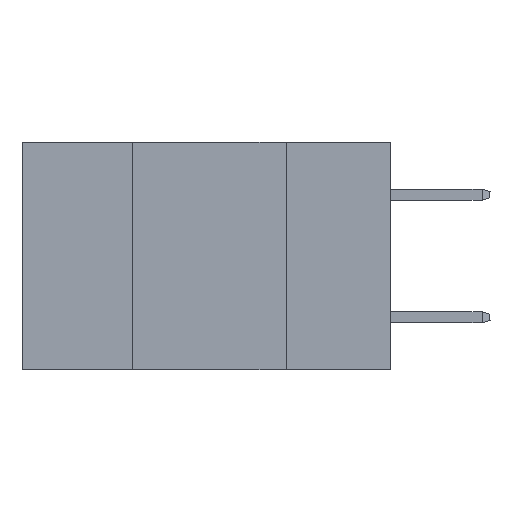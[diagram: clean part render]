
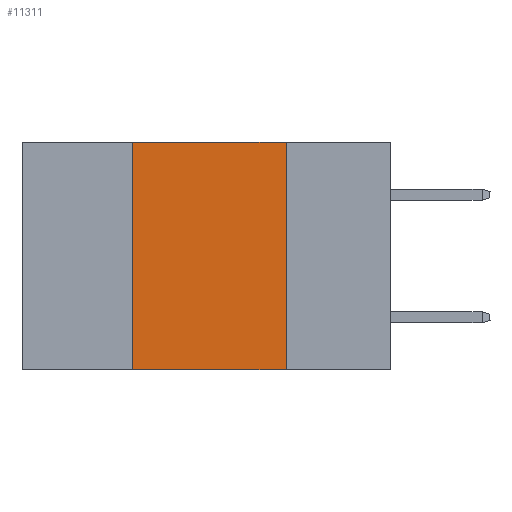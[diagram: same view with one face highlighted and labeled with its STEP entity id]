
A CAD part, left-side view. The second image highlights one B-rep face of the part: STEP entity #11311.
In plain terms, the highlighted planar face has unit normal (-1, 0, 0).
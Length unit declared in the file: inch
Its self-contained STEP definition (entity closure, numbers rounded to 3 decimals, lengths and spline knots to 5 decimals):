
#364 = ORIENTED_EDGE ( 'NONE', *, *, #2774, .F. ) ;
#456 = CARTESIAN_POINT ( 'NONE',  ( 0., 0.6, -0.37 ) ) ;
#1021 = EDGE_CURVE ( 'NONE', #8339, #12660, #4597, .T. ) ;
#1215 = DIRECTION ( 'NONE',  ( 0., 0., -1. ) ) ;
#1250 = EDGE_CURVE ( 'NONE', #8204, #12660, #2606, .T. ) ;
#1634 = CARTESIAN_POINT ( 'NONE',  ( 0., 0.17, 0. ) ) ;
#1653 = DIRECTION ( 'NONE',  ( 0., -1., 0. ) ) ;
#1787 = DIRECTION ( 'NONE',  ( 0., 0., -1. ) ) ;
#2606 = LINE ( 'NONE', #9855, #12658 ) ;
#2774 = EDGE_CURVE ( 'NONE', #8339, #8851, #14405, .T. ) ;
#3448 = ORIENTED_EDGE ( 'NONE', *, *, #7589, .F. ) ;
#3810 = FACE_OUTER_BOUND ( 'NONE', #9949, .T. ) ;
#4597 = LINE ( 'NONE', #456, #9600 ) ;
#6756 = LINE ( 'NONE', #9441, #13606 ) ;
#7075 = AXIS2_PLACEMENT_3D ( 'NONE', #9147, #13721, #1215 ) ;
#7589 = EDGE_CURVE ( 'NONE', #8851, #8204, #6756, .T. ) ;
#8204 = VERTEX_POINT ( 'NONE', #1634 ) ;
#8258 = ORIENTED_EDGE ( 'NONE', *, *, #1250, .F. ) ;
#8339 = VERTEX_POINT ( 'NONE', #11052 ) ;
#8851 = VERTEX_POINT ( 'NONE', #13344 ) ;
#9147 = CARTESIAN_POINT ( 'NONE',  ( 0., 0.6, 0. ) ) ;
#9336 = PLANE ( 'NONE',  #7075 ) ;
#9441 = CARTESIAN_POINT ( 'NONE',  ( 0., 0.6, 0. ) ) ;
#9600 = VECTOR ( 'NONE', #1653, 39.37008 ) ;
#9855 = CARTESIAN_POINT ( 'NONE',  ( 0., 0.17, 0. ) ) ;
#9949 = EDGE_LOOP ( 'NONE', ( #8258, #3448, #364, #14524 ) ) ;
#11052 = CARTESIAN_POINT ( 'NONE',  ( 0., 0.42, -0.37 ) ) ;
#11311 = ADVANCED_FACE ( 'NONE', ( #3810 ), #9336, .F. ) ;
#12043 = VECTOR ( 'NONE', #14620, 39.37008 ) ;
#12349 = CARTESIAN_POINT ( 'NONE',  ( 0., 0.42, 0. ) ) ;
#12658 = VECTOR ( 'NONE', #1787, 39.37008 ) ;
#12660 = VERTEX_POINT ( 'NONE', #14737 ) ;
#13344 = CARTESIAN_POINT ( 'NONE',  ( 0., 0.42, 0. ) ) ;
#13606 = VECTOR ( 'NONE', #14079, 39.37008 ) ;
#13721 = DIRECTION ( 'NONE',  ( 1., 0., 0. ) ) ;
#14079 = DIRECTION ( 'NONE',  ( 0., -1., 0. ) ) ;
#14405 = LINE ( 'NONE', #12349, #12043 ) ;
#14524 = ORIENTED_EDGE ( 'NONE', *, *, #1021, .T. ) ;
#14620 = DIRECTION ( 'NONE',  ( 0., 0., 1. ) ) ;
#14737 = CARTESIAN_POINT ( 'NONE',  ( 0., 0.17, -0.37 ) ) ;
